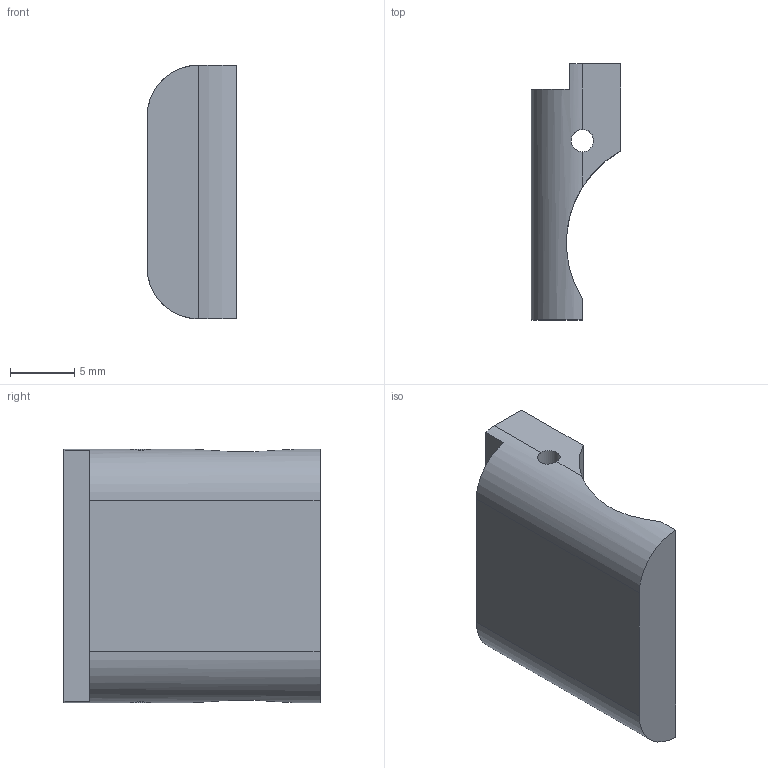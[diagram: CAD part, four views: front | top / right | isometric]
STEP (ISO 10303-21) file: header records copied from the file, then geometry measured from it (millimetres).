
FILE_DESCRIPTION((''),'2;1');
FILE_NAME('PM422FiringPinRetainer1.stp','2015-05-10T23:35:01',('JamesRPatrick'),(''),'Autodesk Inventor 2012','Autodesk Inventor 2012','');
FILE_SCHEMA(('AUTOMOTIVE_DESIGN { 1 0 10303 214 1 1 1 1 }'));
Length unit declared in the file: millimetre
Products named in the file (1): PM422FiringPinRetainer1
Bounding box: 7 x 20 x 19.8 mm (x, y, z)
Volume: 1621.4 mm3; surface area: 1252.2 mm2
Topology: 1 solids, 1 shells, 13 faces, 37 edges, 24 vertices
Faces by surface type: plane 9, cylinder 4
Full cylindrical faces by diameter (mm): 1.75 x1
Entity records: 495 total; most frequent: CARTESIAN_POINT 127, ORIENTED_EDGE 72, DIRECTION 70, EDGE_CURVE 36, AXIS2_PLACEMENT_3D 24, VERTEX_POINT 24, VECTOR 22, LINE 22
